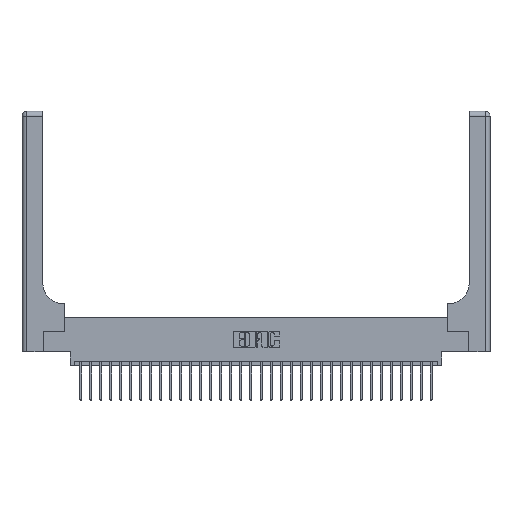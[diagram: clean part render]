
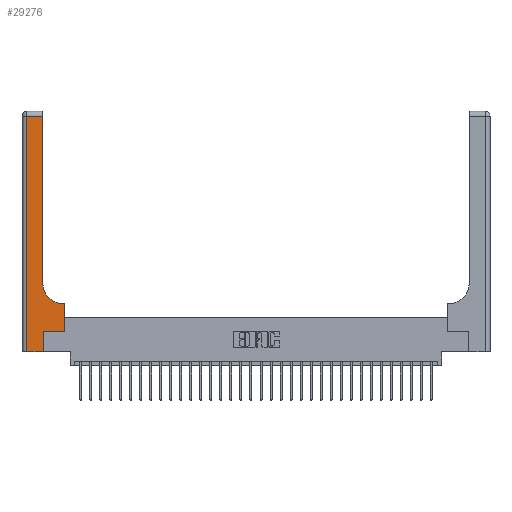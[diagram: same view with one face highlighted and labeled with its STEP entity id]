
A CAD part, top view. The second image highlights one B-rep face of the part: STEP entity #29276.
In plain terms, the highlighted planar face has unit normal (0, 0, 1).
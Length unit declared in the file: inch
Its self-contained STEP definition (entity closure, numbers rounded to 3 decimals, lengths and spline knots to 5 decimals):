
#5 = VECTOR ( 'NONE', #4753, 39.37008 ) ;
#701 = VERTEX_POINT ( 'NONE', #5311 ) ;
#702 = CARTESIAN_POINT ( 'NONE',  ( 0.06, 0., 0.37 ) ) ;
#746 = CARTESIAN_POINT ( 'NONE',  ( 0.26, 2.94, 0.37 ) ) ;
#1035 = VECTOR ( 'NONE', #10538, 39.37008 ) ;
#1105 = DIRECTION ( 'NONE',  ( 1., 0., 0. ) ) ;
#1219 = CARTESIAN_POINT ( 'NONE',  ( 0.26, 3., 0.37 ) ) ;
#1342 = EDGE_CURVE ( 'NONE', #27476, #15752, #6733, .T. ) ;
#1638 = DIRECTION ( 'NONE',  ( -1., 0., 0. ) ) ;
#1937 = CARTESIAN_POINT ( 'NONE',  ( 0., 3., 0.37 ) ) ;
#3400 = LINE ( 'NONE', #21249, #22904 ) ;
#3456 = VECTOR ( 'NONE', #29993, 39.37008 ) ;
#3826 = VERTEX_POINT ( 'NONE', #7725 ) ;
#3928 = DIRECTION ( 'NONE',  ( 0., 0., -1. ) ) ;
#4082 = FACE_OUTER_BOUND ( 'NONE', #26384, .T. ) ;
#4214 = ORIENTED_EDGE ( 'NONE', *, *, #18321, .T. ) ;
#4605 = CARTESIAN_POINT ( 'NONE',  ( 0.528, 0.25, 0.37 ) ) ;
#4753 = DIRECTION ( 'NONE',  ( 0., 1., 0. ) ) ;
#4794 = VERTEX_POINT ( 'NONE', #702 ) ;
#5311 = CARTESIAN_POINT ( 'NONE',  ( 0.265, 0., 0.37 ) ) ;
#5330 = CARTESIAN_POINT ( 'NONE',  ( 0.06, 2.94, 0.37 ) ) ;
#5511 = LINE ( 'NONE', #1219, #1035 ) ;
#5726 = EDGE_CURVE ( 'NONE', #11057, #26469, #5511, .T. ) ;
#6012 = CARTESIAN_POINT ( 'NONE',  ( 0.51, 0.6, 0.37 ) ) ;
#6222 = LINE ( 'NONE', #22224, #22901 ) ;
#6733 = LINE ( 'NONE', #4605, #5 ) ;
#7344 = VERTEX_POINT ( 'NONE', #5330 ) ;
#7725 = CARTESIAN_POINT ( 'NONE',  ( 0.265, 0.25, 0.37 ) ) ;
#8645 = LINE ( 'NONE', #20512, #15464 ) ;
#9151 = AXIS2_PLACEMENT_3D ( 'NONE', #1937, #3928, #25117 ) ;
#9253 = ORIENTED_EDGE ( 'NONE', *, *, #5726, .T. ) ;
#9415 = CARTESIAN_POINT ( 'NONE',  ( 0., 2.94, 0.37 ) ) ;
#10538 = DIRECTION ( 'NONE',  ( 0., 1., 0. ) ) ;
#10606 = ORIENTED_EDGE ( 'NONE', *, *, #15287, .T. ) ;
#11057 = VERTEX_POINT ( 'NONE', #19977 ) ;
#11461 = CARTESIAN_POINT ( 'NONE',  ( 0.265, 0., 0.37 ) ) ;
#11557 = LINE ( 'NONE', #9415, #17363 ) ;
#11729 = ORIENTED_EDGE ( 'NONE', *, *, #18343, .T. ) ;
#12560 = AXIS2_PLACEMENT_3D ( 'NONE', #21532, #24112, #19665 ) ;
#12827 = CARTESIAN_POINT ( 'NONE',  ( 0.528, 0.6, 0.37 ) ) ;
#13255 = LINE ( 'NONE', #22368, #20945 ) ;
#15287 = EDGE_CURVE ( 'NONE', #26469, #7344, #11557, .T. ) ;
#15464 = VECTOR ( 'NONE', #23106, 39.37008 ) ;
#15752 = VERTEX_POINT ( 'NONE', #12827 ) ;
#15969 = ORIENTED_EDGE ( 'NONE', *, *, #19235, .T. ) ;
#16501 = ORIENTED_EDGE ( 'NONE', *, *, #1342, .T. ) ;
#17363 = VECTOR ( 'NONE', #25562, 39.37008 ) ;
#18321 = EDGE_CURVE ( 'NONE', #4794, #701, #13255, .T. ) ;
#18343 = EDGE_CURVE ( 'NONE', #15752, #21159, #6222, .T. ) ;
#19235 = EDGE_CURVE ( 'NONE', #3826, #27476, #3400, .T. ) ;
#19665 = DIRECTION ( 'NONE',  ( 1., 0., 0. ) ) ;
#19967 = CARTESIAN_POINT ( 'NONE',  ( 0.528, 0.25, 0.37 ) ) ;
#19977 = CARTESIAN_POINT ( 'NONE',  ( 0.26, 0.85, 0.37 ) ) ;
#20384 = PLANE ( 'NONE',  #9151 ) ;
#20512 = CARTESIAN_POINT ( 'NONE',  ( 0.06, 3., 0.37 ) ) ;
#20872 = LINE ( 'NONE', #11461, #3456 ) ;
#20945 = VECTOR ( 'NONE', #26930, 39.37008 ) ;
#21067 = EDGE_CURVE ( 'NONE', #701, #3826, #20872, .T. ) ;
#21159 = VERTEX_POINT ( 'NONE', #6012 ) ;
#21249 = CARTESIAN_POINT ( 'NONE',  ( 0.265, 0.25, 0.37 ) ) ;
#21532 = CARTESIAN_POINT ( 'NONE',  ( 0.51, 0.85, 0.37 ) ) ;
#22224 = CARTESIAN_POINT ( 'NONE',  ( 0.26, 0.6, 0.37 ) ) ;
#22368 = CARTESIAN_POINT ( 'NONE',  ( 0., 0., 0.37 ) ) ;
#22408 = ORIENTED_EDGE ( 'NONE', *, *, #27320, .T. ) ;
#22901 = VECTOR ( 'NONE', #1638, 39.37008 ) ;
#22904 = VECTOR ( 'NONE', #1105, 39.37008 ) ;
#23106 = DIRECTION ( 'NONE',  ( 0., -1., 0. ) ) ;
#24112 = DIRECTION ( 'NONE',  ( 0., 0., -1. ) ) ;
#25117 = DIRECTION ( 'NONE',  ( -1., 0., 0. ) ) ;
#25562 = DIRECTION ( 'NONE',  ( -1., 0., 0. ) ) ;
#25689 = CIRCLE ( 'NONE', #12560, 0.25 ) ;
#26384 = EDGE_LOOP ( 'NONE', ( #9253, #10606, #26981, #4214, #29787, #15969, #16501, #11729, #22408 ) ) ;
#26469 = VERTEX_POINT ( 'NONE', #746 ) ;
#26930 = DIRECTION ( 'NONE',  ( 1., 0., 0. ) ) ;
#26981 = ORIENTED_EDGE ( 'NONE', *, *, #28516, .T. ) ;
#27320 = EDGE_CURVE ( 'NONE', #21159, #11057, #25689, .T. ) ;
#27476 = VERTEX_POINT ( 'NONE', #19967 ) ;
#28516 = EDGE_CURVE ( 'NONE', #7344, #4794, #8645, .T. ) ;
#29276 = ADVANCED_FACE ( 'NONE', ( #4082 ), #20384, .F. ) ;
#29787 = ORIENTED_EDGE ( 'NONE', *, *, #21067, .T. ) ;
#29993 = DIRECTION ( 'NONE',  ( 0., 1., 0. ) ) ;
